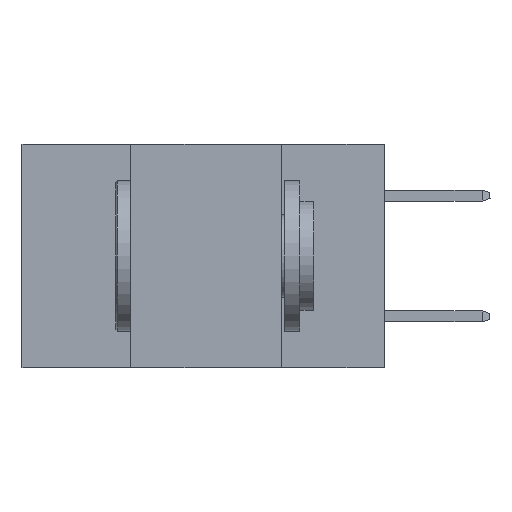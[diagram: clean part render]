
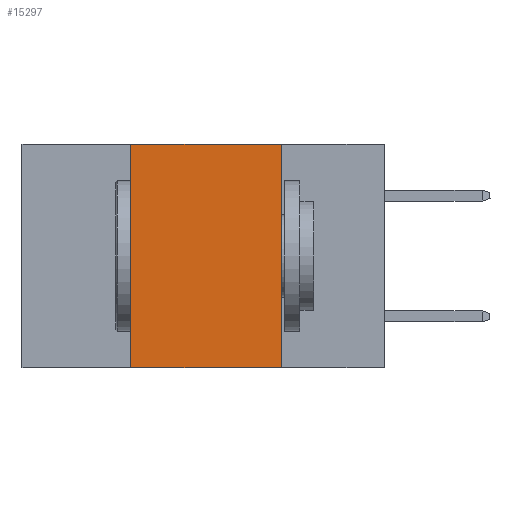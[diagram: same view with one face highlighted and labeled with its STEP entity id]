
A CAD part, left-side view. The second image highlights one B-rep face of the part: STEP entity #15297.
In plain terms, the highlighted planar face has unit normal (-1, 0, 0).
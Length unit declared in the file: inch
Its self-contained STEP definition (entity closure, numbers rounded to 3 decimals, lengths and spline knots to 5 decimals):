
#713 = CARTESIAN_POINT ( 'NONE',  ( 0., 0.17, -0.37 ) ) ;
#855 = VECTOR ( 'NONE', #4079, 39.37008 ) ;
#1106 = PLANE ( 'NONE',  #2424 ) ;
#1219 = DIRECTION ( 'NONE',  ( 1., 0., 0. ) ) ;
#1226 = DIRECTION ( 'NONE',  ( 0., 0., -1. ) ) ;
#1274 = LINE ( 'NONE', #13371, #855 ) ;
#2296 = EDGE_CURVE ( 'NONE', #7882, #13005, #1274, .T. ) ;
#2424 = AXIS2_PLACEMENT_3D ( 'NONE', #10562, #1219, #5139 ) ;
#4009 = EDGE_CURVE ( 'NONE', #5063, #7882, #9776, .T. ) ;
#4079 = DIRECTION ( 'NONE',  ( 0., -1., 0. ) ) ;
#5063 = VERTEX_POINT ( 'NONE', #10381 ) ;
#5139 = DIRECTION ( 'NONE',  ( 0., 0., -1. ) ) ;
#5779 = VECTOR ( 'NONE', #1226, 39.37008 ) ;
#6178 = LINE ( 'NONE', #14432, #5779 ) ;
#7030 = LINE ( 'NONE', #9700, #13056 ) ;
#7863 = EDGE_LOOP ( 'NONE', ( #11754, #9693, #10779, #13098 ) ) ;
#7882 = VERTEX_POINT ( 'NONE', #10552 ) ;
#8809 = FACE_OUTER_BOUND ( 'NONE', #7863, .T. ) ;
#9076 = VERTEX_POINT ( 'NONE', #713 ) ;
#9693 = ORIENTED_EDGE ( 'NONE', *, *, #2296, .F. ) ;
#9700 = CARTESIAN_POINT ( 'NONE',  ( 0., 0.6, -0.37 ) ) ;
#9776 = LINE ( 'NONE', #15884, #15649 ) ;
#10379 = EDGE_CURVE ( 'NONE', #5063, #9076, #7030, .T. ) ;
#10381 = CARTESIAN_POINT ( 'NONE',  ( 0., 0.42, -0.37 ) ) ;
#10552 = CARTESIAN_POINT ( 'NONE',  ( 0., 0.42, 0. ) ) ;
#10562 = CARTESIAN_POINT ( 'NONE',  ( 0., 0.6, 0. ) ) ;
#10779 = ORIENTED_EDGE ( 'NONE', *, *, #4009, .F. ) ;
#10947 = EDGE_CURVE ( 'NONE', #13005, #9076, #6178, .T. ) ;
#11754 = ORIENTED_EDGE ( 'NONE', *, *, #10947, .F. ) ;
#13005 = VERTEX_POINT ( 'NONE', #15462 ) ;
#13056 = VECTOR ( 'NONE', #14317, 39.37008 ) ;
#13098 = ORIENTED_EDGE ( 'NONE', *, *, #10379, .T. ) ;
#13371 = CARTESIAN_POINT ( 'NONE',  ( 0., 0.6, 0. ) ) ;
#14317 = DIRECTION ( 'NONE',  ( 0., -1., 0. ) ) ;
#14432 = CARTESIAN_POINT ( 'NONE',  ( 0., 0.17, 0. ) ) ;
#15297 = ADVANCED_FACE ( 'NONE', ( #8809 ), #1106, .F. ) ;
#15462 = CARTESIAN_POINT ( 'NONE',  ( 0., 0.17, 0. ) ) ;
#15649 = VECTOR ( 'NONE', #17226, 39.37008 ) ;
#15884 = CARTESIAN_POINT ( 'NONE',  ( 0., 0.42, 0. ) ) ;
#17226 = DIRECTION ( 'NONE',  ( 0., 0., 1. ) ) ;
